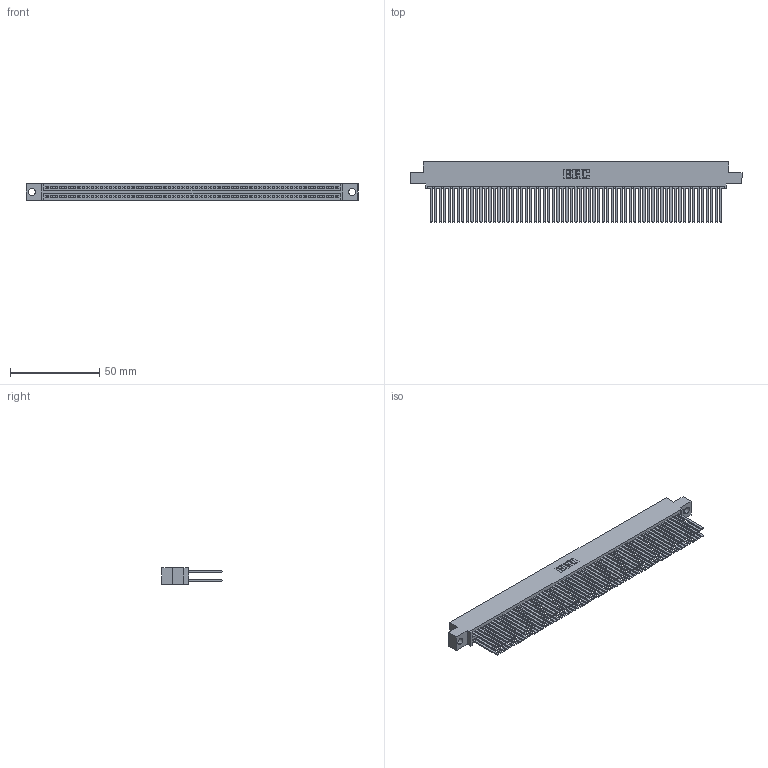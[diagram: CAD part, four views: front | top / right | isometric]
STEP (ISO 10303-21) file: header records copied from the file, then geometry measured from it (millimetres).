
FILE_DESCRIPTION (( 'STEP AP203' ), '1' );
FILE_NAME ('395-130-544-504.STEP', '2021-06-18T00:28:59', ( '' ), ( '' ), 'SwSTEP 2.0', 'SolidWorks 2020', '' );
FILE_SCHEMA (( 'CONFIG_CONTROL_DESIGN' ));
Length unit declared in the file: inch
Products named in the file (3): 345 Part_0.110 Offset - 0.156 Dia-TI; 345-292-001_345-293-144; 395-130-544-504
Assembly tree (131 placements, depth 2):
  395-130-544-504
    345 Part_0.110 Offset - 0.156 Dia-TI
    345-292-001_345-293-144  x130
Bounding box: 186.31 x 33.96 x 9.4 mm (x, y, z)
Volume: 19954.8 mm3; surface area: 35227.6 mm2
Topology: 131 solids, 131 shells, 5864 faces, 17419 edges, 11438 vertices
Faces by surface type: plane 3868, cylinder 1996
Entity records: 48271 total; most frequent: CARTESIAN_POINT 8074, ORIENTED_EDGE 8006, DIRECTION 7087, EDGE_CURVE 4003, LINE 3615, VECTOR 3615, VERTEX_POINT 2666, AXIS2_PLACEMENT_3D 1736
